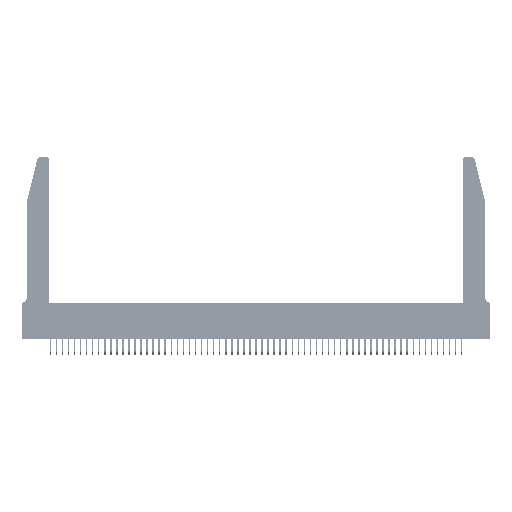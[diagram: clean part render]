
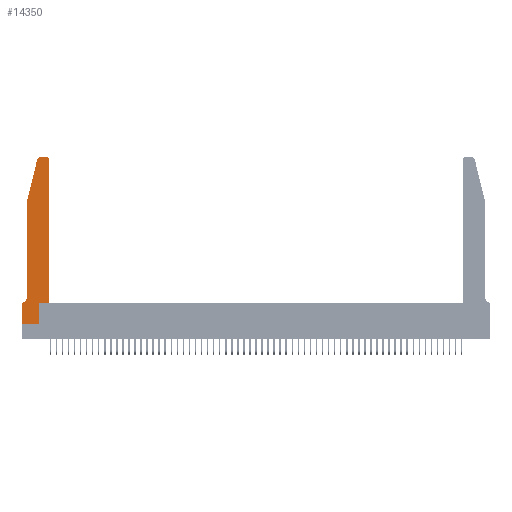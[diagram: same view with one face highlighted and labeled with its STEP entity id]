
A CAD part, top view. The second image highlights one B-rep face of the part: STEP entity #14350.
In plain terms, the highlighted planar face has unit normal (0, 0, 1).
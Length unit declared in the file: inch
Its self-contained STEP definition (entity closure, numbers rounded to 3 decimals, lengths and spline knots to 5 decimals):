
#567 = ORIENTED_EDGE ( 'NONE', *, *, #44055, .T. ) ;
#866 = VERTEX_POINT ( 'NONE', #53484 ) ;
#1002 = VECTOR ( 'NONE', #38513, 39.37008 ) ;
#1360 = CARTESIAN_POINT ( 'NONE',  ( 0.2605, 2.75, 0.37 ) ) ;
#1502 = LINE ( 'NONE', #18492, #22129 ) ;
#1920 = CARTESIAN_POINT ( 'NONE',  ( 0.25487, 2.72718, 0.37 ) ) ;
#2636 = DIRECTION ( 'NONE',  ( 0., 1., 0. ) ) ;
#3269 = DIRECTION ( 'NONE',  ( 0., 0., -1. ) ) ;
#3973 = ORIENTED_EDGE ( 'NONE', *, *, #26843, .T. ) ;
#4243 = DIRECTION ( 'NONE',  ( 0., 0., 1. ) ) ;
#6502 = CARTESIAN_POINT ( 'NONE',  ( 0., 0.35, 0.37 ) ) ;
#7516 = CARTESIAN_POINT ( 'NONE',  ( 0.4205, 2.72, 0.37 ) ) ;
#7669 = VECTOR ( 'NONE', #20355, 39.37008 ) ;
#8039 = ORIENTED_EDGE ( 'NONE', *, *, #53773, .T. ) ;
#8314 = CARTESIAN_POINT ( 'NONE',  ( 0.0755, 0.35, 0.37 ) ) ;
#8788 = LINE ( 'NONE', #17108, #33499 ) ;
#8882 = DIRECTION ( 'NONE',  ( 1., 0., 0. ) ) ;
#10099 = AXIS2_PLACEMENT_3D ( 'NONE', #7516, #21536, #38985 ) ;
#10608 = EDGE_LOOP ( 'NONE', ( #8039, #38004, #53163, #46260, #44132, #50050, #36144, #28394, #35418, #567, #27834, #3973 ) ) ;
#11132 = CARTESIAN_POINT ( 'NONE',  ( 0., 0., 0.37 ) ) ;
#11300 = AXIS2_PLACEMENT_3D ( 'NONE', #11352, #3269, #42435 ) ;
#11352 = CARTESIAN_POINT ( 'NONE',  ( 0.0055, 0.42, 0.37 ) ) ;
#11819 = VERTEX_POINT ( 'NONE', #22223 ) ;
#12330 = DIRECTION ( 'NONE',  ( 0., -1., 0. ) ) ;
#13271 = VERTEX_POINT ( 'NONE', #28879 ) ;
#13310 = CARTESIAN_POINT ( 'NONE',  ( 0.4505, 0.35, 0.37 ) ) ;
#13388 = EDGE_CURVE ( 'NONE', #46350, #11819, #52824, .T. ) ;
#13623 = VECTOR ( 'NONE', #21566, 39.37008 ) ;
#14350 = ADVANCED_FACE ( 'NONE', ( #23161 ), #50338, .T. ) ;
#14724 = LINE ( 'NONE', #32191, #31887 ) ;
#14748 = LINE ( 'NONE', #11132, #1002 ) ;
#15719 = DIRECTION ( 'NONE',  ( 1., 0., 0. ) ) ;
#17108 = CARTESIAN_POINT ( 'NONE',  ( 0., 0., 0.37 ) ) ;
#18128 = LINE ( 'NONE', #37748, #53929 ) ;
#18492 = CARTESIAN_POINT ( 'NONE',  ( 0.0755, 2., 0.37 ) ) ;
#19386 = DIRECTION ( 'NONE',  ( 0., 0., 1. ) ) ;
#20355 = DIRECTION ( 'NONE',  ( 0., 1., 0. ) ) ;
#20623 = EDGE_CURVE ( 'NONE', #26969, #48011, #1502, .T. ) ;
#21521 = VERTEX_POINT ( 'NONE', #37017 ) ;
#21536 = DIRECTION ( 'NONE',  ( 0., 0., 1. ) ) ;
#21566 = DIRECTION ( 'NONE',  ( -1., 0., 0. ) ) ;
#21888 = CARTESIAN_POINT ( 'NONE',  ( 0.284, 2.72, 0.37 ) ) ;
#22129 = VECTOR ( 'NONE', #40944, 39.37008 ) ;
#22223 = CARTESIAN_POINT ( 'NONE',  ( 0., 0.35, 0.37 ) ) ;
#22576 = CARTESIAN_POINT ( 'NONE',  ( 0.2865, 0., 0.37 ) ) ;
#23161 = FACE_OUTER_BOUND ( 'NONE', #10608, .T. ) ;
#23629 = EDGE_CURVE ( 'NONE', #11819, #42944, #8788, .T. ) ;
#24474 = VECTOR ( 'NONE', #8882, 39.37008 ) ;
#25393 = VERTEX_POINT ( 'NONE', #1920 ) ;
#26843 = EDGE_CURVE ( 'NONE', #31302, #31955, #51393, .T. ) ;
#26969 = VERTEX_POINT ( 'NONE', #52088 ) ;
#27834 = ORIENTED_EDGE ( 'NONE', *, *, #45074, .T. ) ;
#28394 = ORIENTED_EDGE ( 'NONE', *, *, #38917, .T. ) ;
#28519 = EDGE_CURVE ( 'NONE', #48011, #46350, #36018, .T. ) ;
#28522 = DIRECTION ( 'NONE',  ( -0.239, -0.971, 0. ) ) ;
#28799 = CARTESIAN_POINT ( 'NONE',  ( 0.2865, 0.35, 0.37 ) ) ;
#28879 = CARTESIAN_POINT ( 'NONE',  ( 0.4505, 0.35, 0.37 ) ) ;
#30617 = LINE ( 'NONE', #13310, #24474 ) ;
#31063 = CARTESIAN_POINT ( 'NONE',  ( 0.4505, 2.72, 0.37 ) ) ;
#31302 = VERTEX_POINT ( 'NONE', #31063 ) ;
#31330 = VECTOR ( 'NONE', #41664, 39.37008 ) ;
#31887 = VECTOR ( 'NONE', #28522, 39.37008 ) ;
#31930 = CARTESIAN_POINT ( 'NONE',  ( 0.4205, 2.75, 0.37 ) ) ;
#31955 = VERTEX_POINT ( 'NONE', #31930 ) ;
#32191 = CARTESIAN_POINT ( 'NONE',  ( 0.0755, 2., 0.37 ) ) ;
#33142 = CARTESIAN_POINT ( 'NONE',  ( 0.0755, 0.42, 0.37 ) ) ;
#33499 = VECTOR ( 'NONE', #12330, 39.37008 ) ;
#33642 = VERTEX_POINT ( 'NONE', #22576 ) ;
#35418 = ORIENTED_EDGE ( 'NONE', *, *, #52064, .T. ) ;
#35539 = AXIS2_PLACEMENT_3D ( 'NONE', #6502, #19386, #15719 ) ;
#36018 = CIRCLE ( 'NONE', #11300, 0.07 ) ;
#36144 = ORIENTED_EDGE ( 'NONE', *, *, #23629, .T. ) ;
#37017 = CARTESIAN_POINT ( 'NONE',  ( 0.2865, 0.35, 0.37 ) ) ;
#37748 = CARTESIAN_POINT ( 'NONE',  ( 0.4505, 0.35, 0.37 ) ) ;
#38004 = ORIENTED_EDGE ( 'NONE', *, *, #44610, .T. ) ;
#38513 = DIRECTION ( 'NONE',  ( 1., 0., 0. ) ) ;
#38917 = EDGE_CURVE ( 'NONE', #42944, #33642, #14748, .T. ) ;
#38985 = DIRECTION ( 'NONE',  ( 1., 0., 0. ) ) ;
#39269 = EDGE_CURVE ( 'NONE', #25393, #26969, #14724, .T. ) ;
#40219 = CARTESIAN_POINT ( 'NONE',  ( 0., 0., 0.37 ) ) ;
#40944 = DIRECTION ( 'NONE',  ( 0., -1., 0. ) ) ;
#41664 = DIRECTION ( 'NONE',  ( -1., 0., 0. ) ) ;
#42435 = DIRECTION ( 'NONE',  ( -1., 0., 0. ) ) ;
#42944 = VERTEX_POINT ( 'NONE', #40219 ) ;
#44055 = EDGE_CURVE ( 'NONE', #21521, #13271, #30617, .T. ) ;
#44132 = ORIENTED_EDGE ( 'NONE', *, *, #28519, .T. ) ;
#44610 = EDGE_CURVE ( 'NONE', #866, #25393, #47783, .T. ) ;
#45074 = EDGE_CURVE ( 'NONE', #13271, #31302, #18128, .T. ) ;
#46260 = ORIENTED_EDGE ( 'NONE', *, *, #20623, .T. ) ;
#46350 = VERTEX_POINT ( 'NONE', #50764 ) ;
#46682 = AXIS2_PLACEMENT_3D ( 'NONE', #21888, #4243, #51873 ) ;
#47783 = CIRCLE ( 'NONE', #46682, 0.03 ) ;
#48011 = VERTEX_POINT ( 'NONE', #33142 ) ;
#49232 = LINE ( 'NONE', #1360, #31330 ) ;
#50050 = ORIENTED_EDGE ( 'NONE', *, *, #13388, .T. ) ;
#50338 = PLANE ( 'NONE',  #35539 ) ;
#50764 = CARTESIAN_POINT ( 'NONE',  ( 0.0055, 0.35, 0.37 ) ) ;
#51393 = CIRCLE ( 'NONE', #10099, 0.03 ) ;
#51873 = DIRECTION ( 'NONE',  ( 1., 0., 0. ) ) ;
#52064 = EDGE_CURVE ( 'NONE', #33642, #21521, #56466, .T. ) ;
#52088 = CARTESIAN_POINT ( 'NONE',  ( 0.0755, 2., 0.37 ) ) ;
#52824 = LINE ( 'NONE', #8314, #13623 ) ;
#53163 = ORIENTED_EDGE ( 'NONE', *, *, #39269, .T. ) ;
#53484 = CARTESIAN_POINT ( 'NONE',  ( 0.284, 2.75, 0.37 ) ) ;
#53773 = EDGE_CURVE ( 'NONE', #31955, #866, #49232, .T. ) ;
#53929 = VECTOR ( 'NONE', #2636, 39.37008 ) ;
#56466 = LINE ( 'NONE', #28799, #7669 ) ;
